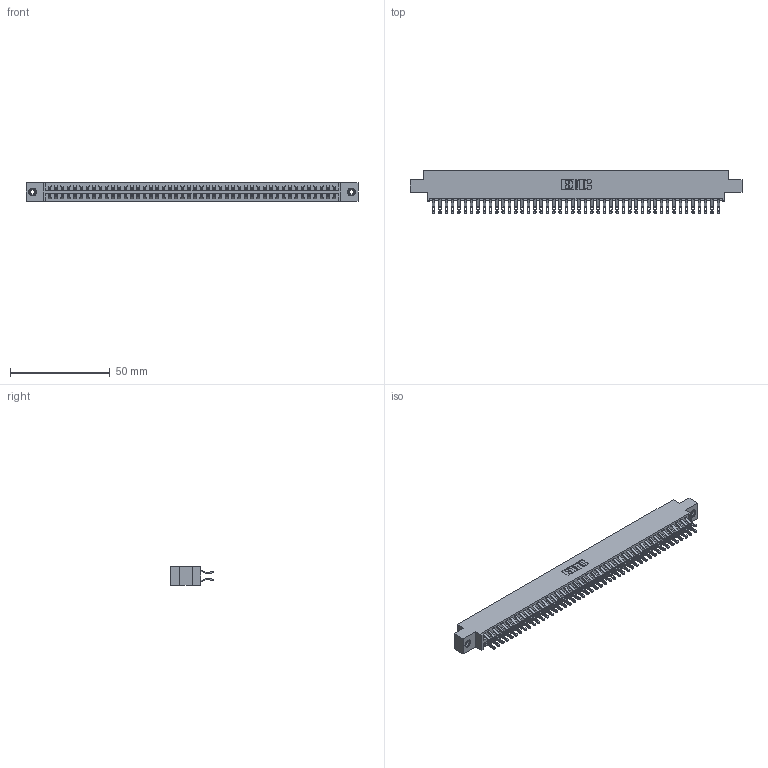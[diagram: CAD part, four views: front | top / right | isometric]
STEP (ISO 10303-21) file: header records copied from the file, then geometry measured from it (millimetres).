
FILE_DESCRIPTION (( 'STEP AP203' ), '1' );
FILE_NAME ('396-092-555-808.STEP', '2019-11-02T16:00:45', ( '' ), ( '' ), 'SwSTEP 2.0', 'SolidWorks 2016', '' );
FILE_SCHEMA (( 'CONFIG_CONTROL_DESIGN' ));
Length unit declared in the file: inch
Products named in the file (4): 346 Part_0.170 Offset - 0.156 Dia-TI; 345-292-001_555 Tail; 345-250-001_345-250-003-102; 396-092-555-808
Assembly tree (95 placements, depth 2):
  396-092-555-808
    346 Part_0.170 Offset - 0.156 Dia-TI
    345-292-001_555 Tail  x92
    345-250-001_345-250-003-102  x2
Bounding box: 166.62 x 21.46 x 9.4 mm (x, y, z)
Volume: 16384.7 mm3; surface area: 23735.6 mm2
Topology: 95 solids, 95 shells, 5522 faces, 17313 edges, 11534 vertices
Faces by surface type: plane 3148, cylinder 2358, cone 12, torus 4
Entity records: 31126 total; most frequent: CARTESIAN_POINT 5145, ORIENTED_EDGE 5042, DIRECTION 4579, EDGE_CURVE 2521, VECTOR 2165, LINE 2165, VERTEX_POINT 1676, AXIS2_PLACEMENT_3D 1207
